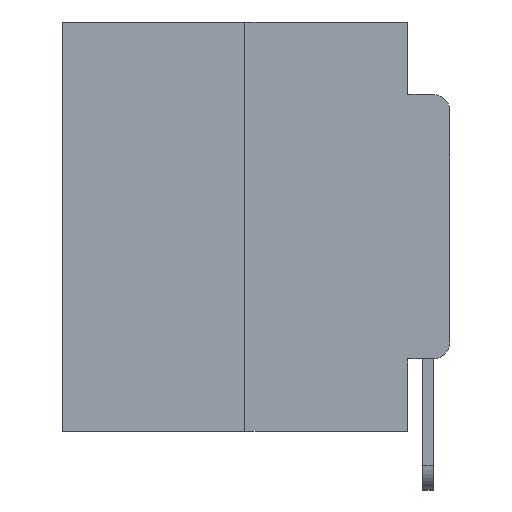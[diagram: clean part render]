
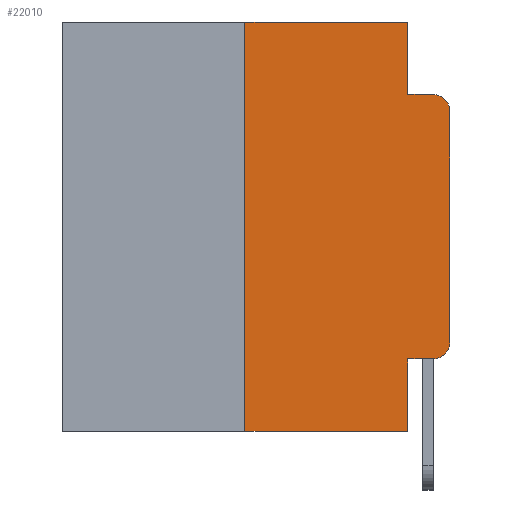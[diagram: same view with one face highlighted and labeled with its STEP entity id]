
A CAD part, left-side view. The second image highlights one B-rep face of the part: STEP entity #22010.
In plain terms, the highlighted planar face has unit normal (-1, 0, 0).
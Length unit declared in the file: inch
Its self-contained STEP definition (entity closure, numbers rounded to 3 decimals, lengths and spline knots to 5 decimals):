
#69 = CARTESIAN_POINT ( 'NONE',  ( 0., 0., -0.1085 ) ) ;
#795 = EDGE_CURVE ( 'NONE', #1873, #820, #9174, .T. ) ;
#797 = LINE ( 'NONE', #20429, #17395 ) ;
#820 = VERTEX_POINT ( 'NONE', #3157 ) ;
#1873 = VERTEX_POINT ( 'NONE', #21822 ) ;
#2257 = DIRECTION ( 'NONE',  ( -1., 0., 0. ) ) ;
#2279 = VERTEX_POINT ( 'NONE', #4047 ) ;
#2769 = AXIS2_PLACEMENT_3D ( 'NONE', #15128, #2257, #17279 ) ;
#3157 = CARTESIAN_POINT ( 'NONE',  ( 0., 0.25, 0. ) ) ;
#4047 = CARTESIAN_POINT ( 'NONE',  ( 0., 0.051, -0.0885 ) ) ;
#4777 = EDGE_CURVE ( 'NONE', #17222, #19697, #23213, .T. ) ;
#5392 = EDGE_CURVE ( 'NONE', #11847, #12250, #14182, .T. ) ;
#5462 = LINE ( 'NONE', #23896, #16043 ) ;
#5682 = DIRECTION ( 'NONE',  ( 0., 0., 1. ) ) ;
#5909 = CARTESIAN_POINT ( 'NONE',  ( 0., 0.473, 0. ) ) ;
#6288 = VECTOR ( 'NONE', #26391, 39.37008 ) ;
#6891 = EDGE_CURVE ( 'NONE', #2279, #12250, #8184, .T. ) ;
#6977 = DIRECTION ( 'NONE',  ( 0., 0., -1. ) ) ;
#7182 = LINE ( 'NONE', #19480, #23406 ) ;
#7591 = ORIENTED_EDGE ( 'NONE', *, *, #795, .F. ) ;
#8184 = LINE ( 'NONE', #21127, #9548 ) ;
#8336 = ORIENTED_EDGE ( 'NONE', *, *, #5392, .T. ) ;
#8432 = LINE ( 'NONE', #5909, #23948 ) ;
#8497 = VECTOR ( 'NONE', #17958, 39.37008 ) ;
#9174 = LINE ( 'NONE', #15885, #8497 ) ;
#9375 = LINE ( 'NONE', #13267, #19872 ) ;
#9548 = VECTOR ( 'NONE', #23267, 39.37008 ) ;
#9643 = EDGE_CURVE ( 'NONE', #820, #12007, #8432, .T. ) ;
#10343 = VERTEX_POINT ( 'NONE', #12035 ) ;
#10618 = EDGE_CURVE ( 'NONE', #19697, #10343, #21904, .T. ) ;
#10684 = EDGE_CURVE ( 'NONE', #17222, #23209, #9375, .T. ) ;
#11263 = ORIENTED_EDGE ( 'NONE', *, *, #9643, .F. ) ;
#11498 = CARTESIAN_POINT ( 'NONE',  ( 0., 0.02, -0.4115 ) ) ;
#11553 = DIRECTION ( 'NONE',  ( -1., 0., 0. ) ) ;
#11642 = CARTESIAN_POINT ( 'NONE',  ( 0., 0.051, -0.5 ) ) ;
#11706 = PLANE ( 'NONE',  #11954 ) ;
#11847 = VERTEX_POINT ( 'NONE', #69 ) ;
#11954 = AXIS2_PLACEMENT_3D ( 'NONE', #24335, #26435, #13746 ) ;
#12007 = VERTEX_POINT ( 'NONE', #19933 ) ;
#12035 = CARTESIAN_POINT ( 'NONE',  ( 0., 0., -0.3915 ) ) ;
#12223 = CARTESIAN_POINT ( 'NONE',  ( 0., 0.02, -0.0885 ) ) ;
#12250 = VERTEX_POINT ( 'NONE', #12223 ) ;
#12363 = DIRECTION ( 'NONE',  ( 0., -1., 0. ) ) ;
#13267 = CARTESIAN_POINT ( 'NONE',  ( 0., 0.051, 0. ) ) ;
#13337 = FACE_OUTER_BOUND ( 'NONE', #17260, .T. ) ;
#13746 = DIRECTION ( 'NONE',  ( 0., 0., -1. ) ) ;
#14182 = CIRCLE ( 'NONE', #25801, 0.02 ) ;
#15128 = CARTESIAN_POINT ( 'NONE',  ( 0., 0.02, -0.3915 ) ) ;
#15885 = CARTESIAN_POINT ( 'NONE',  ( 0., 0.25, 0. ) ) ;
#16043 = VECTOR ( 'NONE', #26015, 39.37008 ) ;
#16419 = ORIENTED_EDGE ( 'NONE', *, *, #10684, .F. ) ;
#16498 = EDGE_CURVE ( 'NONE', #12007, #2279, #5462, .T. ) ;
#17142 = ORIENTED_EDGE ( 'NONE', *, *, #10618, .T. ) ;
#17222 = VERTEX_POINT ( 'NONE', #26242 ) ;
#17260 = EDGE_LOOP ( 'NONE', ( #23864, #8336, #20431, #21800, #11263, #7591, #20780, #16419, #20137, #17142 ) ) ;
#17279 = DIRECTION ( 'NONE',  ( 0., 0., -1. ) ) ;
#17343 = DIRECTION ( 'NONE',  ( 0., -1., 0. ) ) ;
#17395 = VECTOR ( 'NONE', #5682, 39.37008 ) ;
#17958 = DIRECTION ( 'NONE',  ( 0., 0., 1. ) ) ;
#19480 = CARTESIAN_POINT ( 'NONE',  ( 0., 0.473, -0.5 ) ) ;
#19697 = VERTEX_POINT ( 'NONE', #11498 ) ;
#19872 = VECTOR ( 'NONE', #6977, 39.37008 ) ;
#19933 = CARTESIAN_POINT ( 'NONE',  ( 0., 0.051, 0. ) ) ;
#20137 = ORIENTED_EDGE ( 'NONE', *, *, #4777, .T. ) ;
#20429 = CARTESIAN_POINT ( 'NONE',  ( 0., 0., 0. ) ) ;
#20431 = ORIENTED_EDGE ( 'NONE', *, *, #6891, .F. ) ;
#20780 = ORIENTED_EDGE ( 'NONE', *, *, #25500, .T. ) ;
#21127 = CARTESIAN_POINT ( 'NONE',  ( 0., 0.051, -0.0885 ) ) ;
#21800 = ORIENTED_EDGE ( 'NONE', *, *, #16498, .F. ) ;
#21822 = CARTESIAN_POINT ( 'NONE',  ( 0., 0.25, -0.5 ) ) ;
#21904 = CIRCLE ( 'NONE', #2769, 0.02 ) ;
#22010 = ADVANCED_FACE ( 'NONE', ( #13337 ), #11706, .F. ) ;
#22179 = CARTESIAN_POINT ( 'NONE',  ( 0., 0.051, -0.4115 ) ) ;
#23209 = VERTEX_POINT ( 'NONE', #11642 ) ;
#23213 = LINE ( 'NONE', #22179, #6288 ) ;
#23267 = DIRECTION ( 'NONE',  ( 0., -1., 0. ) ) ;
#23406 = VECTOR ( 'NONE', #17343, 39.37008 ) ;
#23864 = ORIENTED_EDGE ( 'NONE', *, *, #25268, .T. ) ;
#23896 = CARTESIAN_POINT ( 'NONE',  ( 0., 0.051, 0. ) ) ;
#23948 = VECTOR ( 'NONE', #12363, 39.37008 ) ;
#24172 = CARTESIAN_POINT ( 'NONE',  ( 0., 0.02, -0.1085 ) ) ;
#24335 = CARTESIAN_POINT ( 'NONE',  ( 0., 0.473, 0. ) ) ;
#25268 = EDGE_CURVE ( 'NONE', #10343, #11847, #797, .T. ) ;
#25500 = EDGE_CURVE ( 'NONE', #1873, #23209, #7182, .T. ) ;
#25801 = AXIS2_PLACEMENT_3D ( 'NONE', #24172, #11553, #26271 ) ;
#26015 = DIRECTION ( 'NONE',  ( 0., 0., -1. ) ) ;
#26242 = CARTESIAN_POINT ( 'NONE',  ( 0., 0.051, -0.4115 ) ) ;
#26271 = DIRECTION ( 'NONE',  ( 0., 0., -1. ) ) ;
#26391 = DIRECTION ( 'NONE',  ( 0., -1., 0. ) ) ;
#26435 = DIRECTION ( 'NONE',  ( 1., 0., 0. ) ) ;
